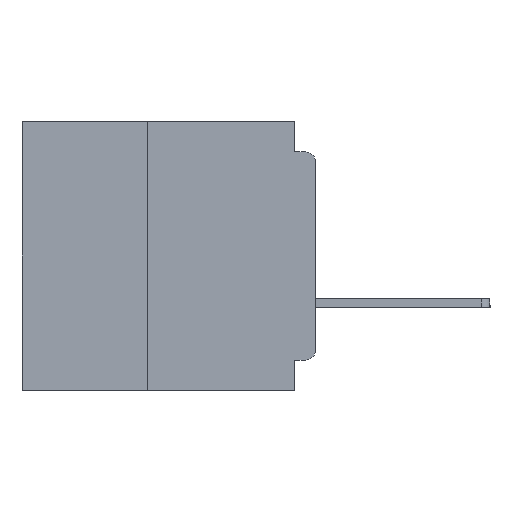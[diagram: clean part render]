
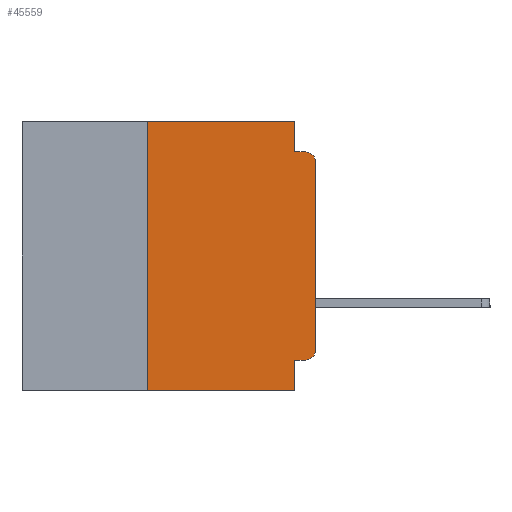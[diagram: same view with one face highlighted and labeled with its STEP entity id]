
A CAD part, left-side view. The second image highlights one B-rep face of the part: STEP entity #45559.
In plain terms, the highlighted planar face has unit normal (-1, 0, 0).
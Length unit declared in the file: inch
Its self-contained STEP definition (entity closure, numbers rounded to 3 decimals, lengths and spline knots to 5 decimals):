
#665 = VECTOR ( 'NONE', #45406, 39.37008 ) ;
#2590 = ORIENTED_EDGE ( 'NONE', *, *, #24268, .T. ) ;
#3215 = VECTOR ( 'NONE', #42821, 39.37008 ) ;
#4579 = ORIENTED_EDGE ( 'NONE', *, *, #47451, .F. ) ;
#4997 = LINE ( 'NONE', #44664, #48286 ) ;
#5279 = CARTESIAN_POINT ( 'NONE',  ( 0., 0.031, 0. ) ) ;
#5465 = EDGE_CURVE ( 'NONE', #18660, #29578, #20947, .T. ) ;
#6323 = CARTESIAN_POINT ( 'NONE',  ( 0., 0.25, -0.4 ) ) ;
#6521 = CARTESIAN_POINT ( 'NONE',  ( 0., 0.25, 0. ) ) ;
#6895 = CARTESIAN_POINT ( 'NONE',  ( 0., 0.25, -0.4 ) ) ;
#7065 = EDGE_CURVE ( 'NONE', #18660, #13446, #52427, .T. ) ;
#7146 = ORIENTED_EDGE ( 'NONE', *, *, #30349, .F. ) ;
#8924 = LINE ( 'NONE', #26933, #29315 ) ;
#9144 = DIRECTION ( 'NONE',  ( 0., 1., 0. ) ) ;
#9413 = ORIENTED_EDGE ( 'NONE', *, *, #35184, .T. ) ;
#9785 = AXIS2_PLACEMENT_3D ( 'NONE', #13525, #17609, #46006 ) ;
#10261 = CARTESIAN_POINT ( 'NONE',  ( 0., 0.015, -0.06 ) ) ;
#10487 = DIRECTION ( 'NONE',  ( 0., 0., 1. ) ) ;
#11625 = LINE ( 'NONE', #12948, #665 ) ;
#12614 = DIRECTION ( 'NONE',  ( -1., 0., 0. ) ) ;
#12948 = CARTESIAN_POINT ( 'NONE',  ( 0., 0.031, -0.4 ) ) ;
#13021 = DIRECTION ( 'NONE',  ( 0., 0., -1. ) ) ;
#13446 = VERTEX_POINT ( 'NONE', #32635 ) ;
#13525 = CARTESIAN_POINT ( 'NONE',  ( 0., 0.437, 0. ) ) ;
#14394 = DIRECTION ( 'NONE',  ( 0., 0., -1. ) ) ;
#14446 = CARTESIAN_POINT ( 'NONE',  ( 0., 0.437, 0. ) ) ;
#16413 = VERTEX_POINT ( 'NONE', #5279 ) ;
#16831 = VECTOR ( 'NONE', #10487, 39.37008 ) ;
#17609 = DIRECTION ( 'NONE',  ( 1., 0., 0. ) ) ;
#17706 = CARTESIAN_POINT ( 'NONE',  ( 0., 0.031, -0.355 ) ) ;
#18660 = VERTEX_POINT ( 'NONE', #18873 ) ;
#18873 = CARTESIAN_POINT ( 'NONE',  ( 0., 0.015, -0.355 ) ) ;
#19284 = FACE_OUTER_BOUND ( 'NONE', #48692, .T. ) ;
#19653 = VECTOR ( 'NONE', #9144, 39.37008 ) ;
#19670 = VERTEX_POINT ( 'NONE', #37968 ) ;
#20440 = LINE ( 'NONE', #39540, #39470 ) ;
#20605 = VERTEX_POINT ( 'NONE', #43364 ) ;
#20947 = LINE ( 'NONE', #21146, #19653 ) ;
#21146 = CARTESIAN_POINT ( 'NONE',  ( 0., 0., -0.355 ) ) ;
#22714 = VECTOR ( 'NONE', #13021, 39.37008 ) ;
#23713 = LINE ( 'NONE', #14446, #3215 ) ;
#24268 = EDGE_CURVE ( 'NONE', #13446, #19670, #4997, .T. ) ;
#26933 = CARTESIAN_POINT ( 'NONE',  ( 0., 0.437, -0.4 ) ) ;
#27761 = ORIENTED_EDGE ( 'NONE', *, *, #39625, .F. ) ;
#28637 = VERTEX_POINT ( 'NONE', #6521 ) ;
#29176 = CARTESIAN_POINT ( 'NONE',  ( 0., 0.031, 0. ) ) ;
#29315 = VECTOR ( 'NONE', #30996, 39.37008 ) ;
#29578 = VERTEX_POINT ( 'NONE', #17706 ) ;
#30166 = AXIS2_PLACEMENT_3D ( 'NONE', #10261, #38709, #14394 ) ;
#30349 = EDGE_CURVE ( 'NONE', #43381, #28637, #37160, .T. ) ;
#30393 = CARTESIAN_POINT ( 'NONE',  ( 0., 0.015, -0.045 ) ) ;
#30996 = DIRECTION ( 'NONE',  ( 0., -1., 0. ) ) ;
#31610 = CARTESIAN_POINT ( 'NONE',  ( 0., 0.031, -0.045 ) ) ;
#31691 = ORIENTED_EDGE ( 'NONE', *, *, #7065, .T. ) ;
#31981 = EDGE_CURVE ( 'NONE', #29578, #20605, #11625, .T. ) ;
#32635 = CARTESIAN_POINT ( 'NONE',  ( 0., 0., -0.34 ) ) ;
#32844 = EDGE_CURVE ( 'NONE', #43381, #20605, #8924, .T. ) ;
#33490 = LINE ( 'NONE', #29176, #22714 ) ;
#34066 = VERTEX_POINT ( 'NONE', #31610 ) ;
#35184 = EDGE_CURVE ( 'NONE', #19670, #40882, #48862, .T. ) ;
#36323 = ORIENTED_EDGE ( 'NONE', *, *, #31981, .F. ) ;
#36966 = CARTESIAN_POINT ( 'NONE',  ( 0., 0.015, -0.34 ) ) ;
#37160 = LINE ( 'NONE', #6323, #16831 ) ;
#37870 = PLANE ( 'NONE',  #9785 ) ;
#37968 = CARTESIAN_POINT ( 'NONE',  ( 0., 0., -0.06 ) ) ;
#38709 = DIRECTION ( 'NONE',  ( -1., 0., 0. ) ) ;
#39470 = VECTOR ( 'NONE', #51553, 39.37008 ) ;
#39540 = CARTESIAN_POINT ( 'NONE',  ( 0., 0., -0.045 ) ) ;
#39625 = EDGE_CURVE ( 'NONE', #28637, #16413, #23713, .T. ) ;
#40882 = VERTEX_POINT ( 'NONE', #30393 ) ;
#40999 = DIRECTION ( 'NONE',  ( 0., 0., -1. ) ) ;
#41249 = ORIENTED_EDGE ( 'NONE', *, *, #5465, .F. ) ;
#42821 = DIRECTION ( 'NONE',  ( 0., -1., 0. ) ) ;
#43253 = ORIENTED_EDGE ( 'NONE', *, *, #50542, .F. ) ;
#43364 = CARTESIAN_POINT ( 'NONE',  ( 0., 0.031, -0.4 ) ) ;
#43381 = VERTEX_POINT ( 'NONE', #6895 ) ;
#44664 = CARTESIAN_POINT ( 'NONE',  ( 0., 0., 0. ) ) ;
#45406 = DIRECTION ( 'NONE',  ( 0., 0., -1. ) ) ;
#45559 = ADVANCED_FACE ( 'NONE', ( #19284 ), #37870, .F. ) ;
#46006 = DIRECTION ( 'NONE',  ( 0., 0., -1. ) ) ;
#47451 = EDGE_CURVE ( 'NONE', #34066, #40882, #20440, .T. ) ;
#48286 = VECTOR ( 'NONE', #48717, 39.37008 ) ;
#48344 = ORIENTED_EDGE ( 'NONE', *, *, #32844, .T. ) ;
#48692 = EDGE_LOOP ( 'NONE', ( #2590, #9413, #4579, #43253, #27761, #7146, #48344, #36323, #41249, #31691 ) ) ;
#48717 = DIRECTION ( 'NONE',  ( 0., 0., 1. ) ) ;
#48862 = CIRCLE ( 'NONE', #30166, 0.015 ) ;
#50542 = EDGE_CURVE ( 'NONE', #16413, #34066, #33490, .T. ) ;
#51229 = AXIS2_PLACEMENT_3D ( 'NONE', #36966, #12614, #40999 ) ;
#51553 = DIRECTION ( 'NONE',  ( 0., -1., 0. ) ) ;
#52427 = CIRCLE ( 'NONE', #51229, 0.015 ) ;
